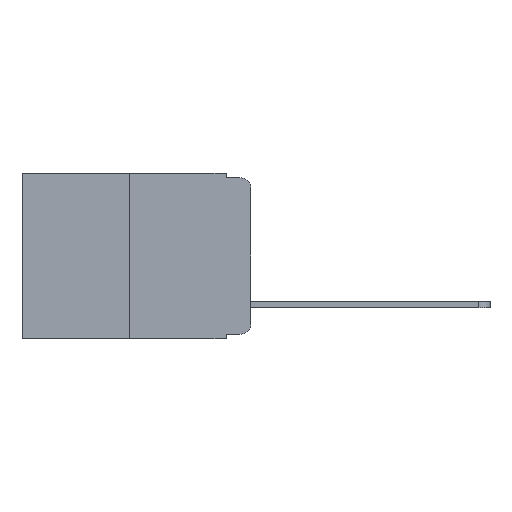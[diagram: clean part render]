
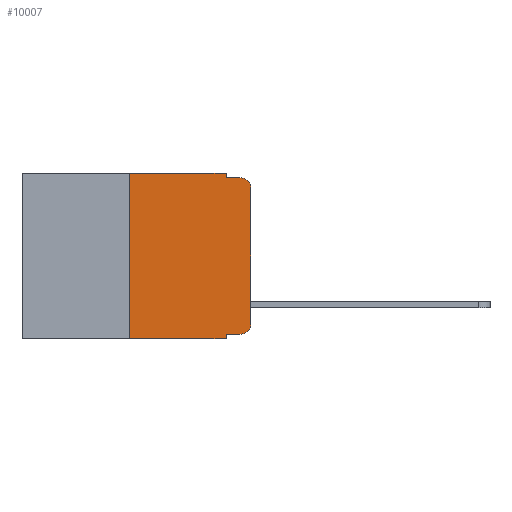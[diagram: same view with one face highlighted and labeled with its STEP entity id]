
A CAD part, left-side view. The second image highlights one B-rep face of the part: STEP entity #10007.
In plain terms, the highlighted planar face has unit normal (-1, 0, 0).
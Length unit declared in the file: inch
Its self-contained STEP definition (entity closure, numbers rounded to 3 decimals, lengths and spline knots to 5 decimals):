
#175 = ORIENTED_EDGE ( 'NONE', *, *, #2302, .F. ) ;
#414 = LINE ( 'NONE', #1321, #6339 ) ;
#590 = VECTOR ( 'NONE', #5217, 39.37008 ) ;
#661 = AXIS2_PLACEMENT_3D ( 'NONE', #10894, #4209, #5082 ) ;
#715 = CARTESIAN_POINT ( 'NONE',  ( 0., 0.25, 0. ) ) ;
#882 = VERTEX_POINT ( 'NONE', #8035 ) ;
#1017 = VERTEX_POINT ( 'NONE', #10425 ) ;
#1069 = DIRECTION ( 'NONE',  ( 0., 0., -1. ) ) ;
#1285 = ORIENTED_EDGE ( 'NONE', *, *, #5547, .T. ) ;
#1291 = DIRECTION ( 'NONE',  ( 0., 0., -1. ) ) ;
#1321 = CARTESIAN_POINT ( 'NONE',  ( 0., 0., 0. ) ) ;
#1347 = VECTOR ( 'NONE', #2537, 39.37008 ) ;
#1557 = DIRECTION ( 'NONE',  ( 0., -1., 0. ) ) ;
#1698 = DIRECTION ( 'NONE',  ( 0., 0., 1. ) ) ;
#1707 = VERTEX_POINT ( 'NONE', #10522 ) ;
#1955 = VERTEX_POINT ( 'NONE', #3404 ) ;
#2093 = CARTESIAN_POINT ( 'NONE',  ( 0., 0.02, -0.01 ) ) ;
#2302 = EDGE_CURVE ( 'NONE', #1707, #7959, #9629, .T. ) ;
#2513 = EDGE_CURVE ( 'NONE', #7421, #1955, #8754, .T. ) ;
#2537 = DIRECTION ( 'NONE',  ( 0., -1., 0. ) ) ;
#3404 = CARTESIAN_POINT ( 'NONE',  ( 0., 0.051, 0. ) ) ;
#3586 = EDGE_CURVE ( 'NONE', #1707, #3743, #5025, .T. ) ;
#3743 = VERTEX_POINT ( 'NONE', #7239 ) ;
#3842 = ORIENTED_EDGE ( 'NONE', *, *, #9172, .T. ) ;
#4037 = CARTESIAN_POINT ( 'NONE',  ( 0., 0.473, 0. ) ) ;
#4139 = CARTESIAN_POINT ( 'NONE',  ( 0., 0.051, -0.333 ) ) ;
#4209 = DIRECTION ( 'NONE',  ( -1., 0., 0. ) ) ;
#4287 = EDGE_LOOP ( 'NONE', ( #3842, #1285, #9464, #7272, #9053, #8051, #11180, #175, #4705, #11533 ) ) ;
#4339 = CARTESIAN_POINT ( 'NONE',  ( 0., 0.473, -0.343 ) ) ;
#4533 = LINE ( 'NONE', #11927, #8077 ) ;
#4588 = EDGE_CURVE ( 'NONE', #3743, #882, #5608, .T. ) ;
#4705 = ORIENTED_EDGE ( 'NONE', *, *, #3586, .T. ) ;
#4737 = EDGE_CURVE ( 'NONE', #12012, #6226, #4533, .T. ) ;
#4882 = CARTESIAN_POINT ( 'NONE',  ( 0., 0.051, 0. ) ) ;
#5025 = LINE ( 'NONE', #4139, #590 ) ;
#5082 = DIRECTION ( 'NONE',  ( 0., 0., -1. ) ) ;
#5135 = FACE_OUTER_BOUND ( 'NONE', #4287, .T. ) ;
#5137 = VERTEX_POINT ( 'NONE', #9371 ) ;
#5217 = DIRECTION ( 'NONE',  ( 0., -1., 0. ) ) ;
#5227 = CARTESIAN_POINT ( 'NONE',  ( 0., 0.051, -0.01 ) ) ;
#5547 = EDGE_CURVE ( 'NONE', #5137, #6226, #9103, .T. ) ;
#5608 = CIRCLE ( 'NONE', #661, 0.02 ) ;
#5868 = EDGE_CURVE ( 'NONE', #1017, #7421, #11318, .T. ) ;
#5921 = PLANE ( 'NONE',  #7298 ) ;
#6072 = DIRECTION ( 'NONE',  ( -1., 0., 0. ) ) ;
#6141 = CARTESIAN_POINT ( 'NONE',  ( 0., 0.02, -0.03 ) ) ;
#6226 = VERTEX_POINT ( 'NONE', #2093 ) ;
#6339 = VECTOR ( 'NONE', #7865, 39.37008 ) ;
#6592 = VECTOR ( 'NONE', #1698, 39.37008 ) ;
#6686 = VECTOR ( 'NONE', #10473, 39.37008 ) ;
#6971 = EDGE_CURVE ( 'NONE', #1017, #7959, #9498, .T. ) ;
#7092 = VECTOR ( 'NONE', #7734, 39.37008 ) ;
#7239 = CARTESIAN_POINT ( 'NONE',  ( 0., 0.02, -0.333 ) ) ;
#7265 = EDGE_CURVE ( 'NONE', #1955, #12012, #9036, .T. ) ;
#7272 = ORIENTED_EDGE ( 'NONE', *, *, #7265, .F. ) ;
#7298 = AXIS2_PLACEMENT_3D ( 'NONE', #4037, #10650, #1069 ) ;
#7421 = VERTEX_POINT ( 'NONE', #11576 ) ;
#7734 = DIRECTION ( 'NONE',  ( 0., 0., -1. ) ) ;
#7744 = CARTESIAN_POINT ( 'NONE',  ( 0., 0.051, 0. ) ) ;
#7865 = DIRECTION ( 'NONE',  ( 0., 0., 1. ) ) ;
#7959 = VERTEX_POINT ( 'NONE', #7961 ) ;
#7961 = CARTESIAN_POINT ( 'NONE',  ( 0., 0.051, -0.343 ) ) ;
#8035 = CARTESIAN_POINT ( 'NONE',  ( 0., 0., -0.313 ) ) ;
#8051 = ORIENTED_EDGE ( 'NONE', *, *, #5868, .F. ) ;
#8064 = DIRECTION ( 'NONE',  ( 0., -1., 0. ) ) ;
#8077 = VECTOR ( 'NONE', #1557, 39.37008 ) ;
#8754 = LINE ( 'NONE', #11051, #1347 ) ;
#9036 = LINE ( 'NONE', #7744, #6686 ) ;
#9053 = ORIENTED_EDGE ( 'NONE', *, *, #2513, .F. ) ;
#9103 = CIRCLE ( 'NONE', #9300, 0.02 ) ;
#9172 = EDGE_CURVE ( 'NONE', #882, #5137, #414, .T. ) ;
#9300 = AXIS2_PLACEMENT_3D ( 'NONE', #6141, #6072, #1291 ) ;
#9371 = CARTESIAN_POINT ( 'NONE',  ( 0., 0., -0.03 ) ) ;
#9464 = ORIENTED_EDGE ( 'NONE', *, *, #4737, .F. ) ;
#9498 = LINE ( 'NONE', #4339, #11851 ) ;
#9629 = LINE ( 'NONE', #4882, #7092 ) ;
#10007 = ADVANCED_FACE ( 'NONE', ( #5135 ), #5921, .F. ) ;
#10425 = CARTESIAN_POINT ( 'NONE',  ( 0., 0.25, -0.343 ) ) ;
#10473 = DIRECTION ( 'NONE',  ( 0., 0., -1. ) ) ;
#10522 = CARTESIAN_POINT ( 'NONE',  ( 0., 0.051, -0.333 ) ) ;
#10650 = DIRECTION ( 'NONE',  ( 1., 0., 0. ) ) ;
#10894 = CARTESIAN_POINT ( 'NONE',  ( 0., 0.02, -0.313 ) ) ;
#11051 = CARTESIAN_POINT ( 'NONE',  ( 0., 0.473, 0. ) ) ;
#11180 = ORIENTED_EDGE ( 'NONE', *, *, #6971, .T. ) ;
#11318 = LINE ( 'NONE', #715, #6592 ) ;
#11533 = ORIENTED_EDGE ( 'NONE', *, *, #4588, .T. ) ;
#11576 = CARTESIAN_POINT ( 'NONE',  ( 0., 0.25, 0. ) ) ;
#11851 = VECTOR ( 'NONE', #8064, 39.37008 ) ;
#11927 = CARTESIAN_POINT ( 'NONE',  ( 0., 0.051, -0.01 ) ) ;
#12012 = VERTEX_POINT ( 'NONE', #5227 ) ;
